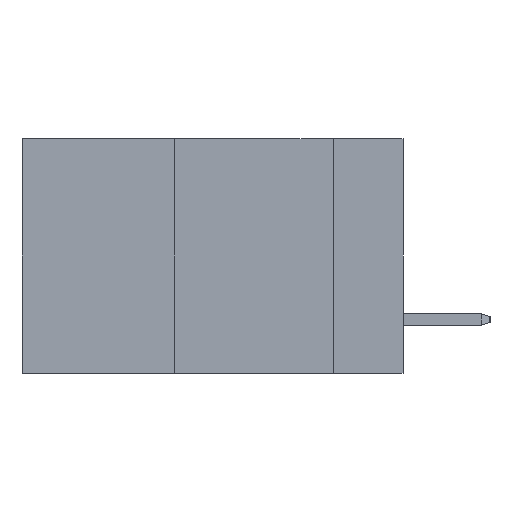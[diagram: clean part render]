
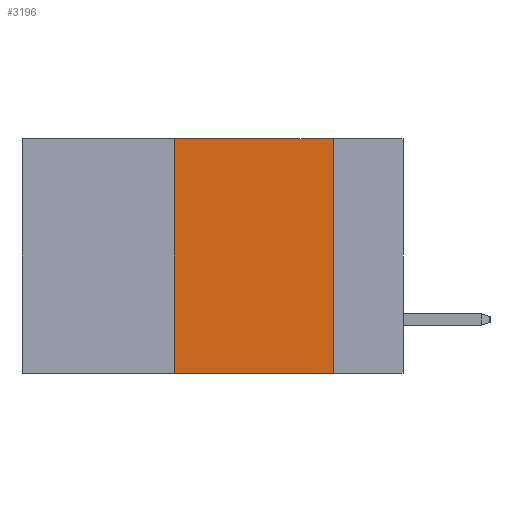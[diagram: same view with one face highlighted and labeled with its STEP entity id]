
A CAD part, left-side view. The second image highlights one B-rep face of the part: STEP entity #3196.
In plain terms, the highlighted planar face has unit normal (-1, 0, 0).
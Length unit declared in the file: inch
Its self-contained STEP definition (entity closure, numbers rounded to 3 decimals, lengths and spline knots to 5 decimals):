
#469 = CARTESIAN_POINT ( 'NONE',  ( 0., 0.36, 0. ) ) ;
#698 = VERTEX_POINT ( 'NONE', #3040 ) ;
#1037 = DIRECTION ( 'NONE',  ( 0., 0., 1. ) ) ;
#1139 = CARTESIAN_POINT ( 'NONE',  ( 0., 0.6, 0. ) ) ;
#1489 = EDGE_CURVE ( 'NONE', #13939, #8614, #2981, .T. ) ;
#1749 = CARTESIAN_POINT ( 'NONE',  ( 0., 0.6, -0.37 ) ) ;
#2238 = AXIS2_PLACEMENT_3D ( 'NONE', #1139, #11084, #6016 ) ;
#2456 = FACE_OUTER_BOUND ( 'NONE', #3496, .T. ) ;
#2981 = LINE ( 'NONE', #1749, #3505 ) ;
#3040 = CARTESIAN_POINT ( 'NONE',  ( 0., 0.11, 0. ) ) ;
#3113 = LINE ( 'NONE', #15420, #12466 ) ;
#3196 = ADVANCED_FACE ( 'NONE', ( #2456 ), #11157, .F. ) ;
#3496 = EDGE_LOOP ( 'NONE', ( #6115, #14164, #8983, #10285 ) ) ;
#3505 = VECTOR ( 'NONE', #9020, 39.37008 ) ;
#3587 = EDGE_CURVE ( 'NONE', #13939, #8254, #4752, .T. ) ;
#4232 = VECTOR ( 'NONE', #8905, 39.37008 ) ;
#4752 = LINE ( 'NONE', #7319, #7149 ) ;
#4943 = LINE ( 'NONE', #6430, #4232 ) ;
#6016 = DIRECTION ( 'NONE',  ( 0., 0., -1. ) ) ;
#6115 = ORIENTED_EDGE ( 'NONE', *, *, #15715, .F. ) ;
#6430 = CARTESIAN_POINT ( 'NONE',  ( 0., 0.6, 0. ) ) ;
#6749 = DIRECTION ( 'NONE',  ( 0., 0., -1. ) ) ;
#7149 = VECTOR ( 'NONE', #1037, 39.37008 ) ;
#7319 = CARTESIAN_POINT ( 'NONE',  ( 0., 0.36, 0. ) ) ;
#8254 = VERTEX_POINT ( 'NONE', #469 ) ;
#8614 = VERTEX_POINT ( 'NONE', #9117 ) ;
#8905 = DIRECTION ( 'NONE',  ( 0., -1., 0. ) ) ;
#8983 = ORIENTED_EDGE ( 'NONE', *, *, #3587, .F. ) ;
#9020 = DIRECTION ( 'NONE',  ( 0., -1., 0. ) ) ;
#9117 = CARTESIAN_POINT ( 'NONE',  ( 0., 0.11, -0.37 ) ) ;
#9993 = CARTESIAN_POINT ( 'NONE',  ( 0., 0.36, -0.37 ) ) ;
#10285 = ORIENTED_EDGE ( 'NONE', *, *, #1489, .T. ) ;
#11084 = DIRECTION ( 'NONE',  ( 1., 0., 0. ) ) ;
#11157 = PLANE ( 'NONE',  #2238 ) ;
#12466 = VECTOR ( 'NONE', #6749, 39.37008 ) ;
#13939 = VERTEX_POINT ( 'NONE', #9993 ) ;
#14164 = ORIENTED_EDGE ( 'NONE', *, *, #15635, .F. ) ;
#15420 = CARTESIAN_POINT ( 'NONE',  ( 0., 0.11, 0. ) ) ;
#15635 = EDGE_CURVE ( 'NONE', #8254, #698, #4943, .T. ) ;
#15715 = EDGE_CURVE ( 'NONE', #698, #8614, #3113, .T. ) ;
